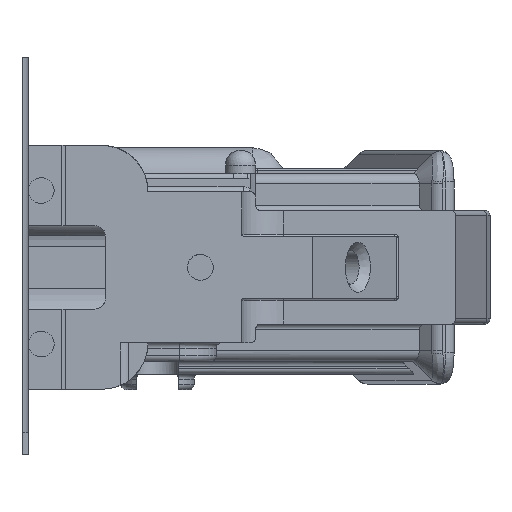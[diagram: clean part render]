
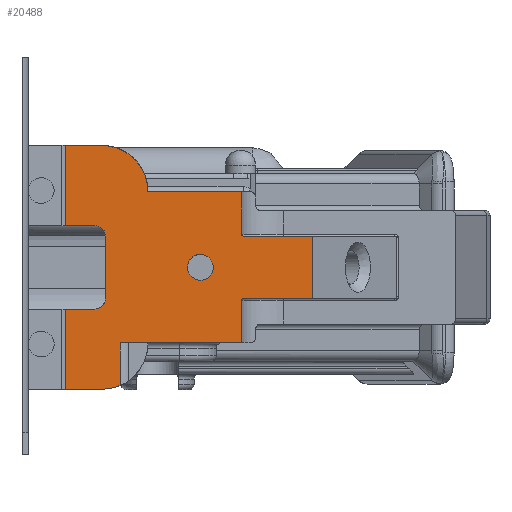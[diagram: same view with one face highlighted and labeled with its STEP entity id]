
A CAD part, left-side view. The second image highlights one B-rep face of the part: STEP entity #20488.
In plain terms, the highlighted planar face has unit normal (-1, 0, 0).
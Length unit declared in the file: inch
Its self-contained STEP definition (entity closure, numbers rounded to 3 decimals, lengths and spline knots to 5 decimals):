
#350=FACE_BOUND('',#3026,.T.);
#1115=PLANE('',#21766);
#1830=FACE_OUTER_BOUND('',#3025,.T.);
#3025=EDGE_LOOP('',(#14910,#14911,#14912,#14913,#14914,#14915,#14916,#14917,
#14918,#14919,#14920,#14921,#14922,#14923,#14924,#14925,#14926,#14927,#14928,
#14929,#14930));
#3026=EDGE_LOOP('',(#14931));
#4451=LINE('',#29179,#6618);
#4540=LINE('',#29524,#6707);
#4672=LINE('',#30071,#6839);
#4674=LINE('',#30077,#6841);
#4675=LINE('',#30081,#6842);
#4681=LINE('',#30094,#6848);
#4687=LINE('',#30112,#6854);
#4688=LINE('',#30117,#6855);
#4689=LINE('',#30119,#6856);
#4690=LINE('',#30121,#6857);
#4691=LINE('',#30125,#6858);
#4692=LINE('',#30127,#6859);
#4693=LINE('',#30129,#6860);
#4694=LINE('',#30133,#6861);
#4695=LINE('',#30135,#6862);
#6618=VECTOR('',#23338,0.47716);
#6707=VECTOR('',#23431,0.4375);
#6839=VECTOR('',#23767,0.3937);
#6841=VECTOR('',#23773,0.3937);
#6842=VECTOR('',#23778,0.47716);
#6848=VECTOR('',#23788,0.4375);
#6854=VECTOR('',#23804,0.375);
#6855=VECTOR('',#23809,0.3937);
#6856=VECTOR('',#23810,0.3937);
#6857=VECTOR('',#23811,0.25563);
#6858=VECTOR('',#23814,0.41801);
#6859=VECTOR('',#23815,0.375);
#6860=VECTOR('',#23816,0.41801);
#6861=VECTOR('',#23819,0.25563);
#6862=VECTOR('',#23820,0.561);
#8571=CIRCLE('',#21767,0.0625);
#8572=CIRCLE('',#21768,0.0625);
#8573=CIRCLE('',#21769,0.27784);
#8574=CIRCLE('',#21770,0.01);
#8575=CIRCLE('',#21771,0.01);
#8576=CIRCLE('',#21772,0.27784);
#8577=CIRCLE('',#21773,0.0775);
#9177=VERTEX_POINT('',#29176);
#9178=VERTEX_POINT('',#29178);
#9299=VERTEX_POINT('',#29521);
#9300=VERTEX_POINT('',#29523);
#9446=VERTEX_POINT('',#30070);
#9448=VERTEX_POINT('',#30076);
#9449=VERTEX_POINT('',#30080);
#9454=VERTEX_POINT('',#30093);
#9460=VERTEX_POINT('',#30109);
#9461=VERTEX_POINT('',#30111);
#9462=VERTEX_POINT('',#30114);
#9463=VERTEX_POINT('',#30116);
#9464=VERTEX_POINT('',#30118);
#9465=VERTEX_POINT('',#30120);
#9466=VERTEX_POINT('',#30122);
#9467=VERTEX_POINT('',#30124);
#9468=VERTEX_POINT('',#30126);
#9469=VERTEX_POINT('',#30128);
#9470=VERTEX_POINT('',#30130);
#9471=VERTEX_POINT('',#30132);
#9472=VERTEX_POINT('',#30134);
#9473=VERTEX_POINT('',#30137);
#11265=EDGE_CURVE('',#9177,#9178,#4451,.T.);
#11388=EDGE_CURVE('',#9299,#9300,#4540,.T.);
#11587=EDGE_CURVE('',#9446,#9178,#4672,.T.);
#11590=EDGE_CURVE('',#9448,#9300,#4674,.T.);
#11592=EDGE_CURVE('',#9448,#9449,#4675,.T.);
#11599=EDGE_CURVE('',#9446,#9454,#4681,.T.);
#11607=EDGE_CURVE('',#9460,#9299,#8571,.T.);
#11608=EDGE_CURVE('',#9461,#9460,#4687,.T.);
#11609=EDGE_CURVE('',#9454,#9461,#8572,.T.);
#11610=EDGE_CURVE('',#9462,#9177,#8573,.T.);
#11611=EDGE_CURVE('',#9462,#9463,#4688,.T.);
#11612=EDGE_CURVE('',#9463,#9464,#4689,.T.);
#11613=EDGE_CURVE('',#9465,#9464,#4690,.T.);
#11614=EDGE_CURVE('',#9466,#9465,#8574,.T.);
#11615=EDGE_CURVE('',#9467,#9466,#4691,.T.);
#11616=EDGE_CURVE('',#9468,#9467,#4692,.T.);
#11617=EDGE_CURVE('',#9469,#9468,#4693,.T.);
#11618=EDGE_CURVE('',#9470,#9469,#8575,.T.);
#11619=EDGE_CURVE('',#9471,#9470,#4694,.T.);
#11620=EDGE_CURVE('',#9472,#9471,#4695,.T.);
#11621=EDGE_CURVE('',#9449,#9472,#8576,.T.);
#11622=EDGE_CURVE('',#9473,#9473,#8577,.T.);
#14910=ORIENTED_EDGE('',*,*,#11590,.T.);
#14911=ORIENTED_EDGE('',*,*,#11388,.F.);
#14912=ORIENTED_EDGE('',*,*,#11607,.F.);
#14913=ORIENTED_EDGE('',*,*,#11608,.F.);
#14914=ORIENTED_EDGE('',*,*,#11609,.F.);
#14915=ORIENTED_EDGE('',*,*,#11599,.F.);
#14916=ORIENTED_EDGE('',*,*,#11587,.T.);
#14917=ORIENTED_EDGE('',*,*,#11265,.F.);
#14918=ORIENTED_EDGE('',*,*,#11610,.F.);
#14919=ORIENTED_EDGE('',*,*,#11611,.T.);
#14920=ORIENTED_EDGE('',*,*,#11612,.T.);
#14921=ORIENTED_EDGE('',*,*,#11613,.F.);
#14922=ORIENTED_EDGE('',*,*,#11614,.F.);
#14923=ORIENTED_EDGE('',*,*,#11615,.F.);
#14924=ORIENTED_EDGE('',*,*,#11616,.F.);
#14925=ORIENTED_EDGE('',*,*,#11617,.F.);
#14926=ORIENTED_EDGE('',*,*,#11618,.F.);
#14927=ORIENTED_EDGE('',*,*,#11619,.F.);
#14928=ORIENTED_EDGE('',*,*,#11620,.F.);
#14929=ORIENTED_EDGE('',*,*,#11621,.F.);
#14930=ORIENTED_EDGE('',*,*,#11592,.F.);
#14931=ORIENTED_EDGE('',*,*,#11622,.F.);
#20488=ADVANCED_FACE('',(#1830,#350),#1115,.F.);
#21766=AXIS2_PLACEMENT_3D('',#30108,#23800,#23801);
#21767=AXIS2_PLACEMENT_3D('',#30110,#23802,#23803);
#21768=AXIS2_PLACEMENT_3D('',#30113,#23805,#23806);
#21769=AXIS2_PLACEMENT_3D('',#30115,#23807,#23808);
#21770=AXIS2_PLACEMENT_3D('',#30123,#23812,#23813);
#21771=AXIS2_PLACEMENT_3D('',#30131,#23817,#23818);
#21772=AXIS2_PLACEMENT_3D('',#30136,#23821,#23822);
#21773=AXIS2_PLACEMENT_3D('',#30138,#23823,#23824);
#23338=DIRECTION('',(0.,1.,0.));
#23431=DIRECTION('',(0.,1.,0.));
#23767=DIRECTION('',(0.,0.,-1.));
#23773=DIRECTION('',(0.,0.,-1.));
#23778=DIRECTION('',(0.,-1.,0.));
#23788=DIRECTION('',(0.,-1.,0.));
#23800=DIRECTION('center_axis',(1.,0.,0.));
#23801=DIRECTION('ref_axis',(0.,0.,-1.));
#23802=DIRECTION('center_axis',(-1.,0.,0.));
#23803=DIRECTION('ref_axis',(0.,-1.,0.));
#23804=DIRECTION('',(0.,0.,1.));
#23805=DIRECTION('center_axis',(-1.,0.,0.));
#23806=DIRECTION('ref_axis',(0.,1.,0.));
#23807=DIRECTION('center_axis',(1.,0.,0.));
#23808=DIRECTION('ref_axis',(0.,0.,1.));
#23809=DIRECTION('',(0.,0.,1.));
#23810=DIRECTION('',(0.,-1.,0.));
#23811=DIRECTION('',(0.,0.,-1.));
#23812=DIRECTION('center_axis',(-1.,0.,0.));
#23813=DIRECTION('ref_axis',(0.,1.,0.));
#23814=DIRECTION('',(0.,1.,0.));
#23815=DIRECTION('',(0.,0.,-1.));
#23816=DIRECTION('',(0.,-1.,0.));
#23817=DIRECTION('center_axis',(-1.,0.,0.));
#23818=DIRECTION('ref_axis',(0.,-1.,0.));
#23819=DIRECTION('',(0.,0.,-1.));
#23820=DIRECTION('',(0.,-1.,0.));
#23821=DIRECTION('center_axis',(1.,0.,0.));
#23822=DIRECTION('ref_axis',(0.,0.,1.));
#23823=DIRECTION('center_axis',(-1.,0.,0.));
#23824=DIRECTION('ref_axis',(0.,1.,0.));
#29176=CARTESIAN_POINT('',(-6.25,-0.22666,-0.73097));
#29178=CARTESIAN_POINT('',(-6.25,-0.01069,-0.73097));
#29179=CARTESIAN_POINT('',(-6.25,-0.22666,-0.73097));
#29521=CARTESIAN_POINT('',(-6.25,-0.187,0.25));
#29523=CARTESIAN_POINT('',(-6.25,-0.01069,0.25));
#29524=CARTESIAN_POINT('',(-6.25,-0.187,0.25));
#30070=CARTESIAN_POINT('',(-6.25,-0.01069,-0.25));
#30071=CARTESIAN_POINT('',(-6.25,-0.01069,0.73097));
#30076=CARTESIAN_POINT('',(-6.25,-0.01069,0.73097));
#30077=CARTESIAN_POINT('',(-6.25,-0.01069,0.73097));
#30080=CARTESIAN_POINT('',(-6.25,-0.22666,0.73097));
#30081=CARTESIAN_POINT('',(-6.25,0.2505,0.73097));
#30093=CARTESIAN_POINT('',(-6.25,-0.187,-0.25));
#30094=CARTESIAN_POINT('',(-6.25,0.2505,-0.25));
#30108=CARTESIAN_POINT('Origin',(-6.25,-0.5805,0.01254));
#30109=CARTESIAN_POINT('',(-6.25,-0.2495,0.1875));
#30110=CARTESIAN_POINT('Origin',(-6.25,-0.187,0.1875));
#30111=CARTESIAN_POINT('',(-6.25,-0.2495,-0.1875));
#30112=CARTESIAN_POINT('',(-6.25,-0.2495,-0.1875));
#30113=CARTESIAN_POINT('Origin',(-6.25,-0.187,-0.1875));
#30114=CARTESIAN_POINT('',(-6.25,-0.3375,-0.7079));
#30115=CARTESIAN_POINT('Origin',(-6.25,-0.22666,-0.45313));
#30116=CARTESIAN_POINT('',(-6.25,-0.3375,-0.45313));
#30117=CARTESIAN_POINT('',(-6.25,-0.3375,-0.34037));
#30118=CARTESIAN_POINT('',(-6.25,-1.0655,-0.45313));
#30119=CARTESIAN_POINT('',(-6.25,-0.509,-0.45313));
#30120=CARTESIAN_POINT('',(-6.25,-1.0655,-0.1975));
#30121=CARTESIAN_POINT('',(-6.25,-1.0655,-0.1975));
#30122=CARTESIAN_POINT('',(-6.25,-1.0755,-0.1875));
#30123=CARTESIAN_POINT('Origin',(-6.25,-1.0755,-0.1975));
#30124=CARTESIAN_POINT('',(-6.25,-1.49351,-0.1875));
#30125=CARTESIAN_POINT('',(-6.25,-1.49351,-0.1875));
#30126=CARTESIAN_POINT('',(-6.25,-1.49351,0.1875));
#30127=CARTESIAN_POINT('',(-6.25,-1.49351,0.1875));
#30128=CARTESIAN_POINT('',(-6.25,-1.0755,0.1875));
#30129=CARTESIAN_POINT('',(-6.25,-1.0755,0.1875));
#30130=CARTESIAN_POINT('',(-6.25,-1.0655,0.1975));
#30131=CARTESIAN_POINT('Origin',(-6.25,-1.0755,0.1975));
#30132=CARTESIAN_POINT('',(-6.25,-1.0655,0.45313));
#30133=CARTESIAN_POINT('',(-6.25,-1.0655,0.45313));
#30134=CARTESIAN_POINT('',(-6.25,-0.5045,0.45313));
#30135=CARTESIAN_POINT('',(-6.25,-0.5045,0.45313));
#30136=CARTESIAN_POINT('Origin',(-6.25,-0.22666,0.45313));
#30137=CARTESIAN_POINT('',(-6.25,-0.897,0.));
#30138=CARTESIAN_POINT('Origin',(-6.25,-0.8195,0.));
